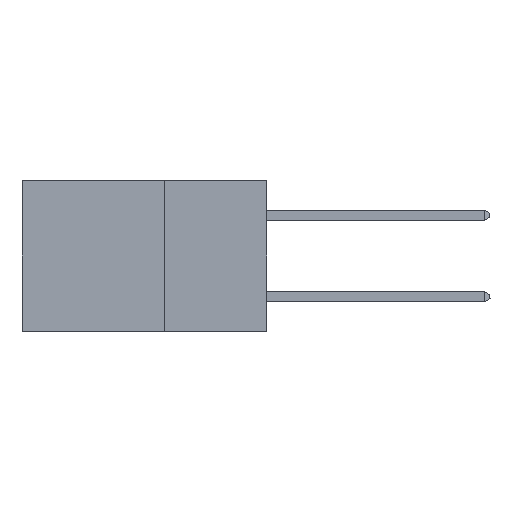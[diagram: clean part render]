
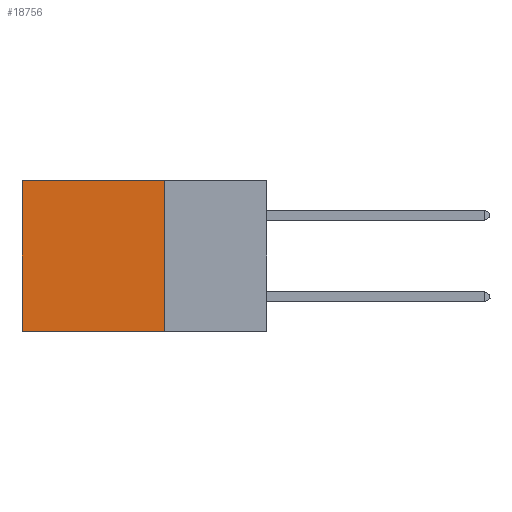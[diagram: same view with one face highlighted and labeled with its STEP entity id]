
A CAD part, left-side view. The second image highlights one B-rep face of the part: STEP entity #18756.
In plain terms, the highlighted planar face has unit normal (-1, 0, 0).
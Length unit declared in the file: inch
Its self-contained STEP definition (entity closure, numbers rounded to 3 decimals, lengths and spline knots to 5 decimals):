
#86 = CARTESIAN_POINT ( 'NONE',  ( 0.2875, 0.6, 0. ) ) ;
#327 = VECTOR ( 'NONE', #12174, 39.37008 ) ;
#3434 = EDGE_LOOP ( 'NONE', ( #16219, #16328, #17547, #18260 ) ) ;
#4790 = LINE ( 'NONE', #13053, #14814 ) ;
#4848 = DIRECTION ( 'NONE',  ( 0., 0., -1. ) ) ;
#5351 = CARTESIAN_POINT ( 'NONE',  ( 0.2875, 0.25, 0. ) ) ;
#7726 = EDGE_CURVE ( 'NONE', #13068, #14713, #10048, .T. ) ;
#8396 = CARTESIAN_POINT ( 'NONE',  ( 0.2875, 0.25, -0.37 ) ) ;
#8603 = EDGE_CURVE ( 'NONE', #9311, #13068, #12801, .T. ) ;
#8965 = LINE ( 'NONE', #9063, #327 ) ;
#9063 = CARTESIAN_POINT ( 'NONE',  ( 0.2875, 0.6, 0. ) ) ;
#9311 = VERTEX_POINT ( 'NONE', #18657 ) ;
#10048 = LINE ( 'NONE', #8396, #19024 ) ;
#11048 = CARTESIAN_POINT ( 'NONE',  ( 0.2875, 0.25, 0. ) ) ;
#11207 = AXIS2_PLACEMENT_3D ( 'NONE', #5351, #18355, #13007 ) ;
#11371 = VERTEX_POINT ( 'NONE', #86 ) ;
#11585 = CARTESIAN_POINT ( 'NONE',  ( 0.2875, 0.25, -0.37 ) ) ;
#12020 = DIRECTION ( 'NONE',  ( 0., 1., 0. ) ) ;
#12174 = DIRECTION ( 'NONE',  ( 0., 0., -1. ) ) ;
#12380 = EDGE_CURVE ( 'NONE', #11371, #14713, #8965, .T. ) ;
#12801 = LINE ( 'NONE', #11048, #13663 ) ;
#13007 = DIRECTION ( 'NONE',  ( 0., 0., -1. ) ) ;
#13053 = CARTESIAN_POINT ( 'NONE',  ( 0.2875, 0.25, 0. ) ) ;
#13068 = VERTEX_POINT ( 'NONE', #11585 ) ;
#13663 = VECTOR ( 'NONE', #4848, 39.37008 ) ;
#14713 = VERTEX_POINT ( 'NONE', #16148 ) ;
#14772 = FACE_OUTER_BOUND ( 'NONE', #3434, .T. ) ;
#14814 = VECTOR ( 'NONE', #19068, 39.37008 ) ;
#16148 = CARTESIAN_POINT ( 'NONE',  ( 0.2875, 0.6, -0.37 ) ) ;
#16219 = ORIENTED_EDGE ( 'NONE', *, *, #12380, .T. ) ;
#16328 = ORIENTED_EDGE ( 'NONE', *, *, #7726, .F. ) ;
#17547 = ORIENTED_EDGE ( 'NONE', *, *, #8603, .F. ) ;
#17646 = EDGE_CURVE ( 'NONE', #9311, #11371, #4790, .T. ) ;
#18260 = ORIENTED_EDGE ( 'NONE', *, *, #17646, .T. ) ;
#18355 = DIRECTION ( 'NONE',  ( 1., 0., 0. ) ) ;
#18657 = CARTESIAN_POINT ( 'NONE',  ( 0.2875, 0.25, 0. ) ) ;
#18756 = ADVANCED_FACE ( 'NONE', ( #14772 ), #19525, .F. ) ;
#19024 = VECTOR ( 'NONE', #12020, 39.37008 ) ;
#19068 = DIRECTION ( 'NONE',  ( 0., 1., 0. ) ) ;
#19525 = PLANE ( 'NONE',  #11207 ) ;
